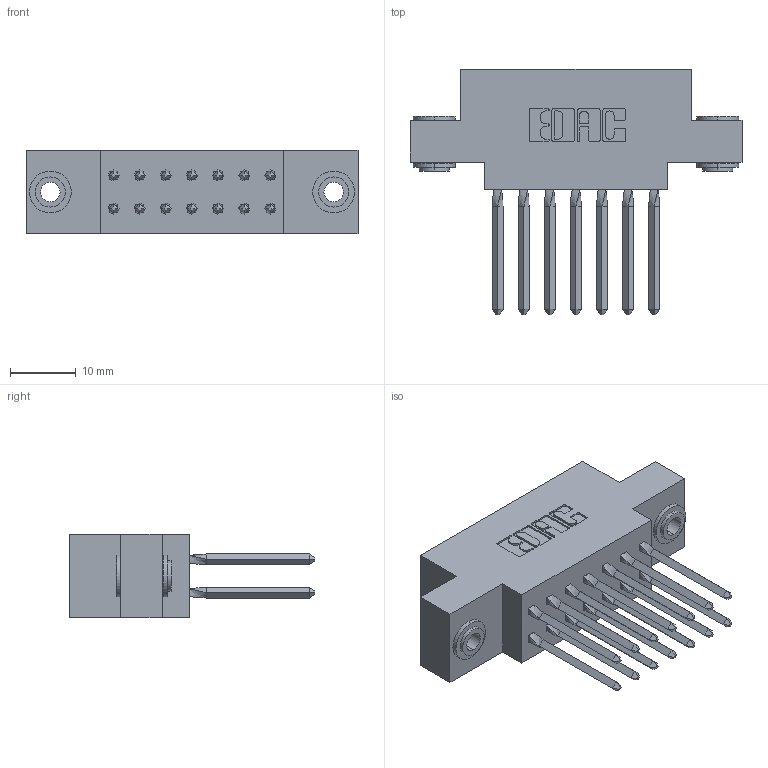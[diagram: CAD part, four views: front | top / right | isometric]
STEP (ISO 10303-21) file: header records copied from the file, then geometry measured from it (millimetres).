
FILE_DESCRIPTION (( 'STEP AP203' ), '1' );
FILE_NAME ('317-014-542-803.STEP', '2020-02-27T14:47:26', ( '' ), ( '' ), 'SwSTEP 2.0', 'SolidWorks 2016', '' );
FILE_SCHEMA (( 'CONFIG_CONTROL_DESIGN' ));
Length unit declared in the file: inch
Products named in the file (4): 317 Part_.156 Dia - TH; 317-290-003_542; 345-250-002_345-250-002-102; 317-014-542-803
Assembly tree (17 placements, depth 2):
  317-014-542-803
    317 Part_.156 Dia - TH
    317-290-003_542  x14
    345-250-002_345-250-002-102  x2
Bounding box: 50.44 x 37.34 x 12.7 mm (x, y, z)
Volume: 7173.4 mm3; surface area: 9068.5 mm2
Topology: 17 solids, 17 shells, 938 faces, 2591 edges, 1658 vertices
Faces by surface type: plane 712, cylinder 162, bspline 56, cone 8
Entity records: 14668 total; most frequent: CARTESIAN_POINT 2772, ORIENTED_EDGE 2428, DIRECTION 2144, EDGE_CURVE 1214, LINE 1020, VECTOR 1020, VERTEX_POINT 802, AXIS2_PLACEMENT_3D 562
